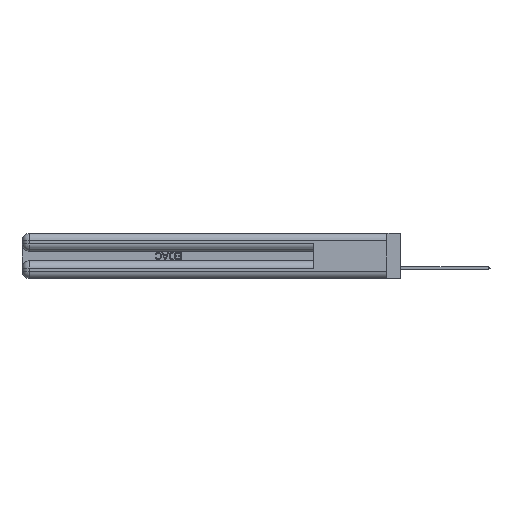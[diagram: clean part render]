
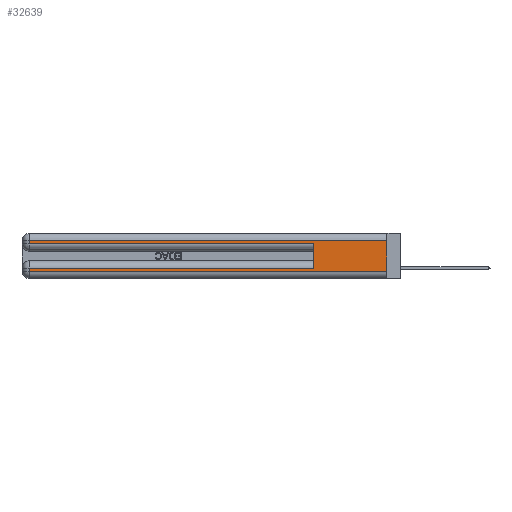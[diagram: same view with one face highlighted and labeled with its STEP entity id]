
A CAD part, left-side view. The second image highlights one B-rep face of the part: STEP entity #32639.
In plain terms, the highlighted planar face has unit normal (-1, 0, 0).
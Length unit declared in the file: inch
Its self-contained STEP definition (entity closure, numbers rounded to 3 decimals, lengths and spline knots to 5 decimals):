
#482 = EDGE_CURVE ( 'NONE', #22356, #48672, #29964, .T. ) ;
#952 = EDGE_LOOP ( 'NONE', ( #13071, #37362, #43189, #34401, #21056, #45211, #3660, #31948 ) ) ;
#1441 = CARTESIAN_POINT ( 'NONE',  ( 0., 2.94, 0.37 ) ) ;
#1487 = LINE ( 'NONE', #43809, #10568 ) ;
#2461 = CARTESIAN_POINT ( 'NONE',  ( 0., 0., 0.37 ) ) ;
#3660 = ORIENTED_EDGE ( 'NONE', *, *, #482, .T. ) ;
#3942 = CARTESIAN_POINT ( 'NONE',  ( 0., 0.6, 0.085 ) ) ;
#5036 = VECTOR ( 'NONE', #35042, 39.37008 ) ;
#5774 = CARTESIAN_POINT ( 'NONE',  ( 0., 0., 0.31 ) ) ;
#6209 = DIRECTION ( 'NONE',  ( 0., -1., 0. ) ) ;
#8076 = CARTESIAN_POINT ( 'NONE',  ( 0., 0., 0.31 ) ) ;
#8839 = EDGE_CURVE ( 'NONE', #49639, #41415, #41323, .T. ) ;
#8840 = VECTOR ( 'NONE', #39369, 39.37008 ) ;
#9310 = VECTOR ( 'NONE', #28604, 39.37008 ) ;
#9652 = DIRECTION ( 'NONE',  ( 1., 0., 0. ) ) ;
#9750 = DIRECTION ( 'NONE',  ( 0., 0., -1. ) ) ;
#10568 = VECTOR ( 'NONE', #31775, 39.37008 ) ;
#11689 = LINE ( 'NONE', #44572, #5036 ) ;
#12298 = CARTESIAN_POINT ( 'NONE',  ( 0., 0.6, 0.285 ) ) ;
#12411 = EDGE_CURVE ( 'NONE', #27186, #30592, #1487, .T. ) ;
#13071 = ORIENTED_EDGE ( 'NONE', *, *, #8839, .F. ) ;
#13184 = EDGE_CURVE ( 'NONE', #48189, #30592, #28132, .T. ) ;
#13461 = EDGE_CURVE ( 'NONE', #48189, #22356, #11689, .T. ) ;
#14660 = FACE_OUTER_BOUND ( 'NONE', #952, .T. ) ;
#15592 = EDGE_CURVE ( 'NONE', #32597, #27186, #38293, .T. ) ;
#17838 = CARTESIAN_POINT ( 'NONE',  ( 0., 2.94, 0.37 ) ) ;
#21056 = ORIENTED_EDGE ( 'NONE', *, *, #13184, .F. ) ;
#22222 = CARTESIAN_POINT ( 'NONE',  ( 0., 2.94, 0.085 ) ) ;
#22356 = VERTEX_POINT ( 'NONE', #22222 ) ;
#23890 = VECTOR ( 'NONE', #6209, 39.37008 ) ;
#24406 = CARTESIAN_POINT ( 'NONE',  ( 0., 2.94, 0.285 ) ) ;
#25886 = DIRECTION ( 'NONE',  ( 0., 0., 1. ) ) ;
#25911 = CARTESIAN_POINT ( 'NONE',  ( 0., 0., 0.06 ) ) ;
#26733 = VECTOR ( 'NONE', #37729, 39.37008 ) ;
#27186 = VERTEX_POINT ( 'NONE', #24406 ) ;
#28132 = LINE ( 'NONE', #41023, #50021 ) ;
#28358 = EDGE_CURVE ( 'NONE', #49639, #32597, #45332, .T. ) ;
#28519 = CARTESIAN_POINT ( 'NONE',  ( 0., 0., 0.06 ) ) ;
#28604 = DIRECTION ( 'NONE',  ( 0., 0., -1. ) ) ;
#28854 = DIRECTION ( 'NONE',  ( 0., 0., -1. ) ) ;
#29142 = AXIS2_PLACEMENT_3D ( 'NONE', #40595, #9652, #28854 ) ;
#29763 = VECTOR ( 'NONE', #9750, 39.37008 ) ;
#29964 = LINE ( 'NONE', #1441, #9310 ) ;
#30592 = VERTEX_POINT ( 'NONE', #12298 ) ;
#31210 = LINE ( 'NONE', #25911, #23890 ) ;
#31775 = DIRECTION ( 'NONE',  ( 0., -1., 0. ) ) ;
#31948 = ORIENTED_EDGE ( 'NONE', *, *, #44982, .T. ) ;
#32597 = VERTEX_POINT ( 'NONE', #46796 ) ;
#32639 = ADVANCED_FACE ( 'NONE', ( #14660 ), #42875, .F. ) ;
#34401 = ORIENTED_EDGE ( 'NONE', *, *, #12411, .T. ) ;
#35042 = DIRECTION ( 'NONE',  ( 0., 1., 0. ) ) ;
#37362 = ORIENTED_EDGE ( 'NONE', *, *, #28358, .T. ) ;
#37729 = DIRECTION ( 'NONE',  ( 0., 0., -1. ) ) ;
#38293 = LINE ( 'NONE', #17838, #26733 ) ;
#39369 = DIRECTION ( 'NONE',  ( 0., 1., 0. ) ) ;
#40595 = CARTESIAN_POINT ( 'NONE',  ( 0., 0., 0.37 ) ) ;
#41023 = CARTESIAN_POINT ( 'NONE',  ( 0., 0.6, 0.145 ) ) ;
#41323 = LINE ( 'NONE', #2461, #29763 ) ;
#41415 = VERTEX_POINT ( 'NONE', #28519 ) ;
#42875 = PLANE ( 'NONE',  #29142 ) ;
#43189 = ORIENTED_EDGE ( 'NONE', *, *, #15592, .T. ) ;
#43809 = CARTESIAN_POINT ( 'NONE',  ( 0., 0., 0.285 ) ) ;
#44572 = CARTESIAN_POINT ( 'NONE',  ( 0., 0., 0.085 ) ) ;
#44982 = EDGE_CURVE ( 'NONE', #48672, #41415, #31210, .T. ) ;
#45211 = ORIENTED_EDGE ( 'NONE', *, *, #13461, .T. ) ;
#45332 = LINE ( 'NONE', #8076, #8840 ) ;
#45651 = CARTESIAN_POINT ( 'NONE',  ( 0., 2.94, 0.06 ) ) ;
#46796 = CARTESIAN_POINT ( 'NONE',  ( 0., 2.94, 0.31 ) ) ;
#48189 = VERTEX_POINT ( 'NONE', #3942 ) ;
#48672 = VERTEX_POINT ( 'NONE', #45651 ) ;
#49639 = VERTEX_POINT ( 'NONE', #5774 ) ;
#50021 = VECTOR ( 'NONE', #25886, 39.37008 ) ;
